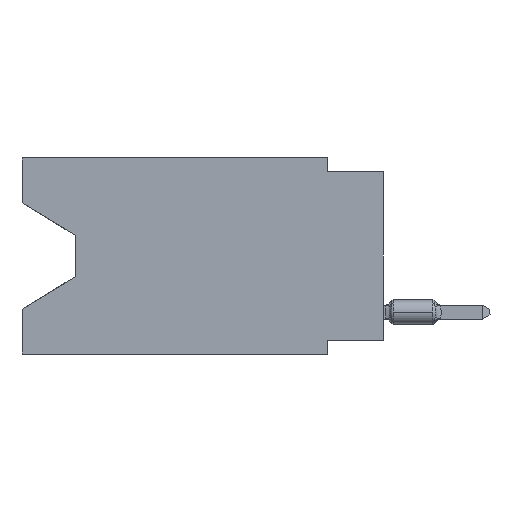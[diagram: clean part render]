
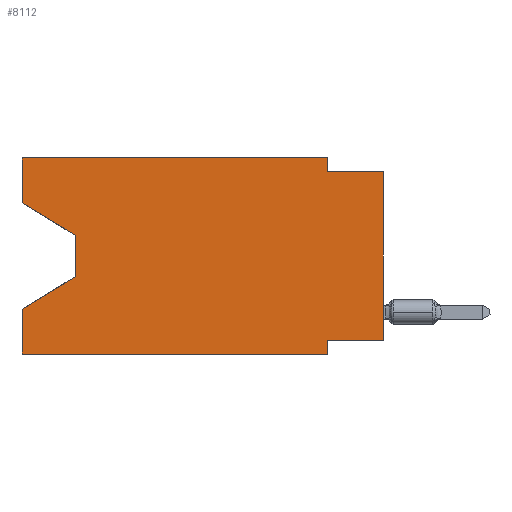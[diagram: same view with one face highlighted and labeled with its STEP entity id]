
A CAD part, left-side view. The second image highlights one B-rep face of the part: STEP entity #8112.
In plain terms, the highlighted planar face has unit normal (-1, 0, 0).
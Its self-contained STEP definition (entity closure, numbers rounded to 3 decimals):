
#139 = FACE_OUTER_BOUND ( 'NONE', #5425, .T. ) ;
#150 = CARTESIAN_POINT ( 'NONE',  ( 0., 0., 0. ) ) ;
#222 = CARTESIAN_POINT ( 'NONE',  ( 0., 16.383, -6.852 ) ) ;
#408 = DIRECTION ( 'NONE',  ( 0., -1., 0. ) ) ;
#413 = CARTESIAN_POINT ( 'NONE',  ( 0., 16.383, -2.038 ) ) ;
#455 = VECTOR ( 'NONE', #14062, 1000. ) ;
#964 = ORIENTED_EDGE ( 'NONE', *, *, #14004, .T. ) ;
#1607 = CARTESIAN_POINT ( 'NONE',  ( 0., 2.54, -0.635 ) ) ;
#1756 = VERTEX_POINT ( 'NONE', #6227 ) ;
#1760 = LINE ( 'NONE', #7085, #455 ) ;
#1818 = CARTESIAN_POINT ( 'NONE',  ( 0., 13.97, -5.385 ) ) ;
#2688 = VECTOR ( 'NONE', #9410, 1000. ) ;
#2773 = VERTEX_POINT ( 'NONE', #222 ) ;
#2852 = EDGE_CURVE ( 'NONE', #3551, #11425, #1760, .T. ) ;
#3193 = EDGE_CURVE ( 'NONE', #6696, #4828, #12849, .T. ) ;
#3275 = CARTESIAN_POINT ( 'NONE',  ( 0., 16.383, 0. ) ) ;
#3295 = CARTESIAN_POINT ( 'NONE',  ( 0., 0., -0.635 ) ) ;
#3333 = VECTOR ( 'NONE', #11228, 1000. ) ;
#3475 = ORIENTED_EDGE ( 'NONE', *, *, #15057, .F. ) ;
#3551 = VERTEX_POINT ( 'NONE', #11197 ) ;
#4061 = CARTESIAN_POINT ( 'NONE',  ( 0., 2.54, -8.89 ) ) ;
#4141 = EDGE_CURVE ( 'NONE', #8918, #11077, #11633, .T. ) ;
#4293 = CARTESIAN_POINT ( 'NONE',  ( 0., 16.383, 0. ) ) ;
#4305 = DIRECTION ( 'NONE',  ( 0., 0., 1. ) ) ;
#4339 = LINE ( 'NONE', #16749, #15636 ) ;
#4774 = DIRECTION ( 'NONE',  ( 0., -1., 0. ) ) ;
#4828 = VERTEX_POINT ( 'NONE', #17822 ) ;
#4955 = DIRECTION ( 'NONE',  ( 0., 0., -1. ) ) ;
#5041 = CARTESIAN_POINT ( 'NONE',  ( 0., 13.97, -3.505 ) ) ;
#5425 = EDGE_LOOP ( 'NONE', ( #13071, #964, #6722, #10083, #8621, #3475, #14560, #9049, #11062, #5729, #16686, #6656 ) ) ;
#5729 = ORIENTED_EDGE ( 'NONE', *, *, #16548, .F. ) ;
#5746 = VECTOR ( 'NONE', #4305, 1000. ) ;
#5755 = VERTEX_POINT ( 'NONE', #11252 ) ;
#5846 = VECTOR ( 'NONE', #14325, 1000. ) ;
#6227 = CARTESIAN_POINT ( 'NONE',  ( 0., 2.54, 0. ) ) ;
#6525 = VECTOR ( 'NONE', #4774, 1000. ) ;
#6656 = ORIENTED_EDGE ( 'NONE', *, *, #14845, .F. ) ;
#6696 = VERTEX_POINT ( 'NONE', #13447 ) ;
#6722 = ORIENTED_EDGE ( 'NONE', *, *, #10315, .T. ) ;
#7029 = LINE ( 'NONE', #15271, #10817 ) ;
#7085 = CARTESIAN_POINT ( 'NONE',  ( 0., 0., -8.255 ) ) ;
#7095 = DIRECTION ( 'NONE',  ( 0., 0., -1. ) ) ;
#7335 = LINE ( 'NONE', #1818, #16716 ) ;
#7883 = CARTESIAN_POINT ( 'NONE',  ( 0., 0., -0.635 ) ) ;
#7938 = LINE ( 'NONE', #5041, #16143 ) ;
#8112 = ADVANCED_FACE ( 'NONE', ( #139 ), #14354, .F. ) ;
#8621 = ORIENTED_EDGE ( 'NONE', *, *, #3193, .T. ) ;
#8918 = VERTEX_POINT ( 'NONE', #1607 ) ;
#9049 = ORIENTED_EDGE ( 'NONE', *, *, #13201, .T. ) ;
#9410 = DIRECTION ( 'NONE',  ( 0., 0., -1. ) ) ;
#9752 = DIRECTION ( 'NONE',  ( 0., 0., -1. ) ) ;
#10083 = ORIENTED_EDGE ( 'NONE', *, *, #11148, .F. ) ;
#10098 = DIRECTION ( 'NONE',  ( 1., 0., 0. ) ) ;
#10157 = LINE ( 'NONE', #3275, #5846 ) ;
#10315 = EDGE_CURVE ( 'NONE', #5755, #2773, #7335, .T. ) ;
#10585 = DIRECTION ( 'NONE',  ( 0., -0.855, -0.519 ) ) ;
#10817 = VECTOR ( 'NONE', #9752, 1000. ) ;
#11062 = ORIENTED_EDGE ( 'NONE', *, *, #4141, .F. ) ;
#11077 = VERTEX_POINT ( 'NONE', #7883 ) ;
#11148 = EDGE_CURVE ( 'NONE', #6696, #2773, #4339, .T. ) ;
#11197 = CARTESIAN_POINT ( 'NONE',  ( 0., 0., -8.255 ) ) ;
#11228 = DIRECTION ( 'NONE',  ( 0., -1., 0. ) ) ;
#11252 = CARTESIAN_POINT ( 'NONE',  ( 0., 13.97, -5.385 ) ) ;
#11425 = VERTEX_POINT ( 'NONE', #17388 ) ;
#11633 = LINE ( 'NONE', #3295, #12047 ) ;
#11863 = LINE ( 'NONE', #17389, #14127 ) ;
#11998 = VERTEX_POINT ( 'NONE', #16675 ) ;
#12047 = VECTOR ( 'NONE', #408, 1000. ) ;
#12545 = LINE ( 'NONE', #150, #5746 ) ;
#12641 = EDGE_CURVE ( 'NONE', #14338, #15341, #11863, .T. ) ;
#12849 = LINE ( 'NONE', #16914, #6525 ) ;
#13071 = ORIENTED_EDGE ( 'NONE', *, *, #12641, .T. ) ;
#13201 = EDGE_CURVE ( 'NONE', #3551, #11077, #12545, .T. ) ;
#13447 = CARTESIAN_POINT ( 'NONE',  ( 0., 16.383, -8.89 ) ) ;
#14004 = EDGE_CURVE ( 'NONE', #15341, #5755, #7938, .T. ) ;
#14062 = DIRECTION ( 'NONE',  ( 0., 1., 0. ) ) ;
#14118 = CARTESIAN_POINT ( 'NONE',  ( 0., 16.383, 0. ) ) ;
#14127 = VECTOR ( 'NONE', #10585, 1000. ) ;
#14325 = DIRECTION ( 'NONE',  ( 0., 0., 1. ) ) ;
#14338 = VERTEX_POINT ( 'NONE', #413 ) ;
#14354 = PLANE ( 'NONE',  #14805 ) ;
#14560 = ORIENTED_EDGE ( 'NONE', *, *, #2852, .F. ) ;
#14805 = AXIS2_PLACEMENT_3D ( 'NONE', #4293, #10098, #7095 ) ;
#14845 = EDGE_CURVE ( 'NONE', #14338, #11998, #10157, .T. ) ;
#15057 = EDGE_CURVE ( 'NONE', #11425, #4828, #16557, .T. ) ;
#15110 = DIRECTION ( 'NONE',  ( 0., 0., 1. ) ) ;
#15271 = CARTESIAN_POINT ( 'NONE',  ( 0., 2.54, 0. ) ) ;
#15341 = VERTEX_POINT ( 'NONE', #17465 ) ;
#15636 = VECTOR ( 'NONE', #15110, 1000. ) ;
#16143 = VECTOR ( 'NONE', #4955, 1000. ) ;
#16548 = EDGE_CURVE ( 'NONE', #1756, #8918, #7029, .T. ) ;
#16557 = LINE ( 'NONE', #4061, #2688 ) ;
#16675 = CARTESIAN_POINT ( 'NONE',  ( 0., 16.383, 0. ) ) ;
#16686 = ORIENTED_EDGE ( 'NONE', *, *, #17718, .F. ) ;
#16716 = VECTOR ( 'NONE', #16752, 1000. ) ;
#16741 = LINE ( 'NONE', #14118, #3333 ) ;
#16749 = CARTESIAN_POINT ( 'NONE',  ( 0., 16.383, 0. ) ) ;
#16752 = DIRECTION ( 'NONE',  ( 0., 0.855, -0.519 ) ) ;
#16914 = CARTESIAN_POINT ( 'NONE',  ( 0., 16.383, -8.89 ) ) ;
#17388 = CARTESIAN_POINT ( 'NONE',  ( 0., 2.54, -8.255 ) ) ;
#17389 = CARTESIAN_POINT ( 'NONE',  ( 0., 16.383, -2.038 ) ) ;
#17465 = CARTESIAN_POINT ( 'NONE',  ( 0., 13.97, -3.505 ) ) ;
#17718 = EDGE_CURVE ( 'NONE', #11998, #1756, #16741, .T. ) ;
#17822 = CARTESIAN_POINT ( 'NONE',  ( 0., 2.54, -8.89 ) ) ;
